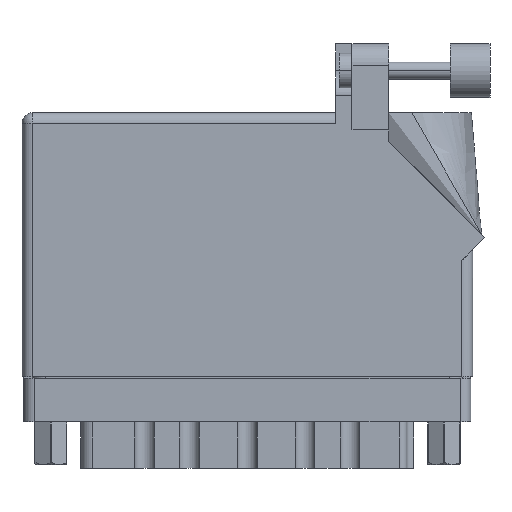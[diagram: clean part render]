
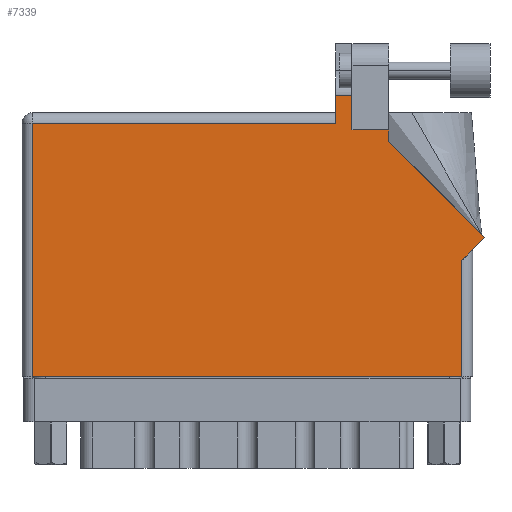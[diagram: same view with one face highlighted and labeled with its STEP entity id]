
A CAD part, front view. The second image highlights one B-rep face of the part: STEP entity #7339.
In plain terms, the highlighted face is planar.
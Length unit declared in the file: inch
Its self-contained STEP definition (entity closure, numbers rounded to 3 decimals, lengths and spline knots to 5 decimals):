
#54 = VERTEX_POINT ( 'NONE', #16194 ) ;
#486 = DIRECTION ( 'NONE',  ( 0.707, 0.707, 0. ) ) ;
#1237 = CARTESIAN_POINT ( 'NONE',  ( 2.68271, 0.80771, 0. ) ) ;
#1457 = EDGE_CURVE ( 'NONE', #37513, #10184, #60859, .T. ) ;
#2131 = CARTESIAN_POINT ( 'NONE',  ( 0.062, 0., 0. ) ) ;
#2608 = LINE ( 'NONE', #21942, #36336 ) ;
#2948 = ORIENTED_EDGE ( 'NONE', *, *, #50927, .T. ) ;
#2964 = CARTESIAN_POINT ( 'NONE',  ( 2.55, 0.675, 0. ) ) ;
#3517 = ORIENTED_EDGE ( 'NONE', *, *, #12359, .T. ) ;
#5660 = DIRECTION ( 'NONE',  ( 0., 1., 0. ) ) ;
#5984 = CARTESIAN_POINT ( 'NONE',  ( 1.913, 1.43, 0. ) ) ;
#6448 = CARTESIAN_POINT ( 'NONE',  ( 2.126, 1.36442, 0. ) ) ;
#6554 = CARTESIAN_POINT ( 'NONE',  ( 2.24377, 1.6315, 0. ) ) ;
#7339 = ADVANCED_FACE ( 'NONE', ( #59656 ), #49539, .F. ) ;
#7914 = CARTESIAN_POINT ( 'NONE',  ( 0., 1.468, 0. ) ) ;
#8387 = ORIENTED_EDGE ( 'NONE', *, *, #19783, .T. ) ;
#8501 = VERTEX_POINT ( 'NONE', #16925 ) ;
#8713 = CARTESIAN_POINT ( 'NONE',  ( 2.126, 1.43, 0. ) ) ;
#10184 = VERTEX_POINT ( 'NONE', #56727 ) ;
#12063 = DIRECTION ( 'NONE',  ( -1., 0., 0. ) ) ;
#12359 = EDGE_CURVE ( 'NONE', #8501, #24488, #17920, .T. ) ;
#13607 = EDGE_CURVE ( 'NONE', #55023, #8501, #49904, .T. ) ;
#16194 = CARTESIAN_POINT ( 'NONE',  ( 2.55, 0., 0. ) ) ;
#16346 = CARTESIAN_POINT ( 'NONE',  ( 2.126, 1.36442, 0. ) ) ;
#16352 = LINE ( 'NONE', #16663, #55016 ) ;
#16576 = DIRECTION ( 'NONE',  ( 0., 1., 0. ) ) ;
#16663 = CARTESIAN_POINT ( 'NONE',  ( 1.913, 1.43, 0. ) ) ;
#16925 = CARTESIAN_POINT ( 'NONE',  ( 2.126, 1.43, 0. ) ) ;
#17920 = LINE ( 'NONE', #8713, #22837 ) ;
#18959 = EDGE_CURVE ( 'NONE', #35556, #54, #2608, .T. ) ;
#19783 = EDGE_CURVE ( 'NONE', #59889, #39954, #30659, .T. ) ;
#20296 = VECTOR ( 'NONE', #36778, 39.37008 ) ;
#20394 = VECTOR ( 'NONE', #60877, 39.37008 ) ;
#20572 = DIRECTION ( 'NONE',  ( -0.707, 0.707, 0. ) ) ;
#20863 = LINE ( 'NONE', #54167, #25409 ) ;
#21942 = CARTESIAN_POINT ( 'NONE',  ( 0., 0., 0. ) ) ;
#22743 = ORIENTED_EDGE ( 'NONE', *, *, #1457, .T. ) ;
#22837 = VECTOR ( 'NONE', #62281, 39.37008 ) ;
#23737 = AXIS2_PLACEMENT_3D ( 'NONE', #25729, #55848, #12063 ) ;
#24488 = VERTEX_POINT ( 'NONE', #5984 ) ;
#24760 = ORIENTED_EDGE ( 'NONE', *, *, #31630, .T. ) ;
#24957 = VECTOR ( 'NONE', #20572, 39.37008 ) ;
#24966 = DIRECTION ( 'NONE',  ( -1., 0., 0. ) ) ;
#25409 = VECTOR ( 'NONE', #5660, 39.37008 ) ;
#25729 = CARTESIAN_POINT ( 'NONE',  ( 0., 1.53, 0. ) ) ;
#25857 = EDGE_LOOP ( 'NONE', ( #2948, #8387, #50522, #22743, #24760, #25947, #50364, #29298, #57408, #41483, #3517 ) ) ;
#25947 = ORIENTED_EDGE ( 'NONE', *, *, #18959, .T. ) ;
#27993 = EDGE_CURVE ( 'NONE', #50396, #29988, #29649, .T. ) ;
#28324 = VECTOR ( 'NONE', #24966, 39.37008 ) ;
#29298 = ORIENTED_EDGE ( 'NONE', *, *, #27993, .T. ) ;
#29649 = LINE ( 'NONE', #39199, #48213 ) ;
#29988 = VERTEX_POINT ( 'NONE', #50803 ) ;
#30538 = CARTESIAN_POINT ( 'NONE',  ( 1.819, 1.468, 0. ) ) ;
#30659 = LINE ( 'NONE', #6554, #28324 ) ;
#31630 = EDGE_CURVE ( 'NONE', #10184, #35556, #34828, .T. ) ;
#34828 = LINE ( 'NONE', #2131, #48333 ) ;
#35257 = CARTESIAN_POINT ( 'NONE',  ( 1.913, 1.6315, 0. ) ) ;
#35556 = VERTEX_POINT ( 'NONE', #51293 ) ;
#36336 = VECTOR ( 'NONE', #41306, 39.37008 ) ;
#36778 = DIRECTION ( 'NONE',  ( -1., 0., 0. ) ) ;
#37513 = VERTEX_POINT ( 'NONE', #30538 ) ;
#39199 = CARTESIAN_POINT ( 'NONE',  ( 2.612, 0.737, 0. ) ) ;
#39908 = DIRECTION ( 'NONE',  ( 0., -1., 0. ) ) ;
#39954 = VERTEX_POINT ( 'NONE', #44410 ) ;
#41306 = DIRECTION ( 'NONE',  ( 1., 0., 0. ) ) ;
#41483 = ORIENTED_EDGE ( 'NONE', *, *, #13607, .T. ) ;
#41554 = CARTESIAN_POINT ( 'NONE',  ( 1.819, 1.53, 0. ) ) ;
#42275 = VECTOR ( 'NONE', #16576, 39.37008 ) ;
#44410 = CARTESIAN_POINT ( 'NONE',  ( 1.819, 1.6315, 0. ) ) ;
#44674 = LINE ( 'NONE', #1237, #24957 ) ;
#46313 = LINE ( 'NONE', #41554, #20394 ) ;
#47043 = EDGE_CURVE ( 'NONE', #39954, #37513, #46313, .T. ) ;
#47257 = EDGE_CURVE ( 'NONE', #54, #50396, #20863, .T. ) ;
#48213 = VECTOR ( 'NONE', #486, 39.37008 ) ;
#48333 = VECTOR ( 'NONE', #39908, 39.37008 ) ;
#49539 = PLANE ( 'NONE',  #23737 ) ;
#49904 = LINE ( 'NONE', #6448, #42275 ) ;
#50364 = ORIENTED_EDGE ( 'NONE', *, *, #47257, .T. ) ;
#50396 = VERTEX_POINT ( 'NONE', #2964 ) ;
#50522 = ORIENTED_EDGE ( 'NONE', *, *, #47043, .T. ) ;
#50594 = DIRECTION ( 'NONE',  ( 0., 1., 0. ) ) ;
#50803 = CARTESIAN_POINT ( 'NONE',  ( 2.68271, 0.80771, 0. ) ) ;
#50927 = EDGE_CURVE ( 'NONE', #24488, #59889, #16352, .T. ) ;
#51293 = CARTESIAN_POINT ( 'NONE',  ( 0.062, 0., 0. ) ) ;
#54167 = CARTESIAN_POINT ( 'NONE',  ( 2.55, 0.737, 0. ) ) ;
#54570 = EDGE_CURVE ( 'NONE', #29988, #55023, #44674, .T. ) ;
#55016 = VECTOR ( 'NONE', #50594, 39.37008 ) ;
#55023 = VERTEX_POINT ( 'NONE', #16346 ) ;
#55848 = DIRECTION ( 'NONE',  ( 0., 0., -1. ) ) ;
#56727 = CARTESIAN_POINT ( 'NONE',  ( 0.062, 1.468, 0. ) ) ;
#57408 = ORIENTED_EDGE ( 'NONE', *, *, #54570, .T. ) ;
#59656 = FACE_OUTER_BOUND ( 'NONE', #25857, .T. ) ;
#59889 = VERTEX_POINT ( 'NONE', #35257 ) ;
#60859 = LINE ( 'NONE', #7914, #20296 ) ;
#60877 = DIRECTION ( 'NONE',  ( 0., -1., 0. ) ) ;
#62281 = DIRECTION ( 'NONE',  ( -1., 0., 0. ) ) ;
